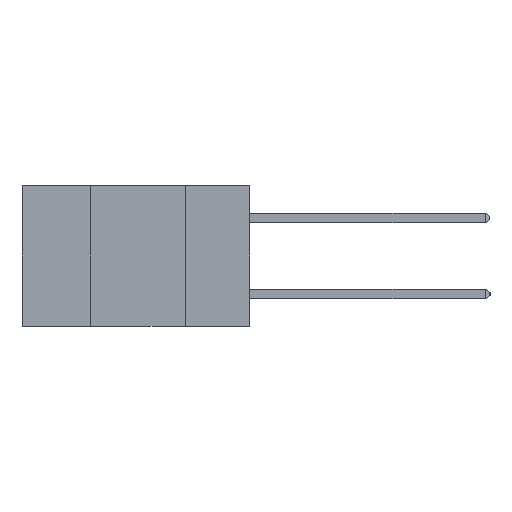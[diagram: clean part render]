
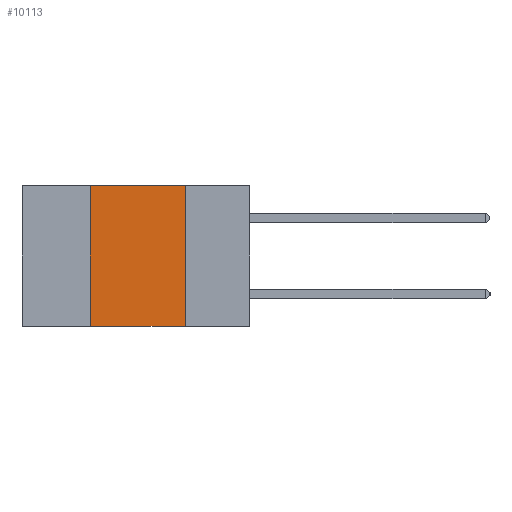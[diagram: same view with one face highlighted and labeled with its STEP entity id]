
A CAD part, left-side view. The second image highlights one B-rep face of the part: STEP entity #10113.
In plain terms, the highlighted planar face has unit normal (-1, 0, 0).
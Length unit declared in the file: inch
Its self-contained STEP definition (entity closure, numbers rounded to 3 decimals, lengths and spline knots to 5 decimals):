
#26 = DIRECTION ( 'NONE',  ( 0., 0., -1. ) ) ;
#499 = EDGE_LOOP ( 'NONE', ( #4795, #12311, #5794, #2300 ) ) ;
#1000 = LINE ( 'NONE', #8903, #11050 ) ;
#1054 = FACE_OUTER_BOUND ( 'NONE', #499, .T. ) ;
#1137 = EDGE_CURVE ( 'NONE', #2352, #13195, #1000, .T. ) ;
#2008 = CARTESIAN_POINT ( 'NONE',  ( 0., 0.17, 0. ) ) ;
#2300 = ORIENTED_EDGE ( 'NONE', *, *, #7683, .T. ) ;
#2352 = VERTEX_POINT ( 'NONE', #12706 ) ;
#3089 = VERTEX_POINT ( 'NONE', #10199 ) ;
#3420 = VERTEX_POINT ( 'NONE', #11786 ) ;
#3861 = DIRECTION ( 'NONE',  ( 0., -1., 0. ) ) ;
#4544 = LINE ( 'NONE', #6454, #7573 ) ;
#4795 = ORIENTED_EDGE ( 'NONE', *, *, #5404, .F. ) ;
#5404 = EDGE_CURVE ( 'NONE', #13195, #3089, #9404, .T. ) ;
#5794 = ORIENTED_EDGE ( 'NONE', *, *, #8850, .F. ) ;
#6454 = CARTESIAN_POINT ( 'NONE',  ( 0., 0.6, -0.37 ) ) ;
#6710 = PLANE ( 'NONE',  #7660 ) ;
#6767 = DIRECTION ( 'NONE',  ( 0., 0., -1. ) ) ;
#6938 = VECTOR ( 'NONE', #16614, 39.37008 ) ;
#7249 = CARTESIAN_POINT ( 'NONE',  ( 0., 0.17, 0. ) ) ;
#7573 = VECTOR ( 'NONE', #3861, 39.37008 ) ;
#7660 = AXIS2_PLACEMENT_3D ( 'NONE', #15698, #7970, #26 ) ;
#7683 = EDGE_CURVE ( 'NONE', #3420, #3089, #4544, .T. ) ;
#7970 = DIRECTION ( 'NONE',  ( 1., 0., 0. ) ) ;
#8850 = EDGE_CURVE ( 'NONE', #3420, #2352, #12573, .T. ) ;
#8903 = CARTESIAN_POINT ( 'NONE',  ( 0., 0.6, 0. ) ) ;
#8912 = CARTESIAN_POINT ( 'NONE',  ( 0., 0.42, 0. ) ) ;
#9013 = VECTOR ( 'NONE', #6767, 39.37008 ) ;
#9404 = LINE ( 'NONE', #2008, #9013 ) ;
#10113 = ADVANCED_FACE ( 'NONE', ( #1054 ), #6710, .F. ) ;
#10199 = CARTESIAN_POINT ( 'NONE',  ( 0., 0.17, -0.37 ) ) ;
#11050 = VECTOR ( 'NONE', #14958, 39.37008 ) ;
#11786 = CARTESIAN_POINT ( 'NONE',  ( 0., 0.42, -0.37 ) ) ;
#12311 = ORIENTED_EDGE ( 'NONE', *, *, #1137, .F. ) ;
#12573 = LINE ( 'NONE', #8912, #6938 ) ;
#12706 = CARTESIAN_POINT ( 'NONE',  ( 0., 0.42, 0. ) ) ;
#13195 = VERTEX_POINT ( 'NONE', #7249 ) ;
#14958 = DIRECTION ( 'NONE',  ( 0., -1., 0. ) ) ;
#15698 = CARTESIAN_POINT ( 'NONE',  ( 0., 0.6, 0. ) ) ;
#16614 = DIRECTION ( 'NONE',  ( 0., 0., 1. ) ) ;
